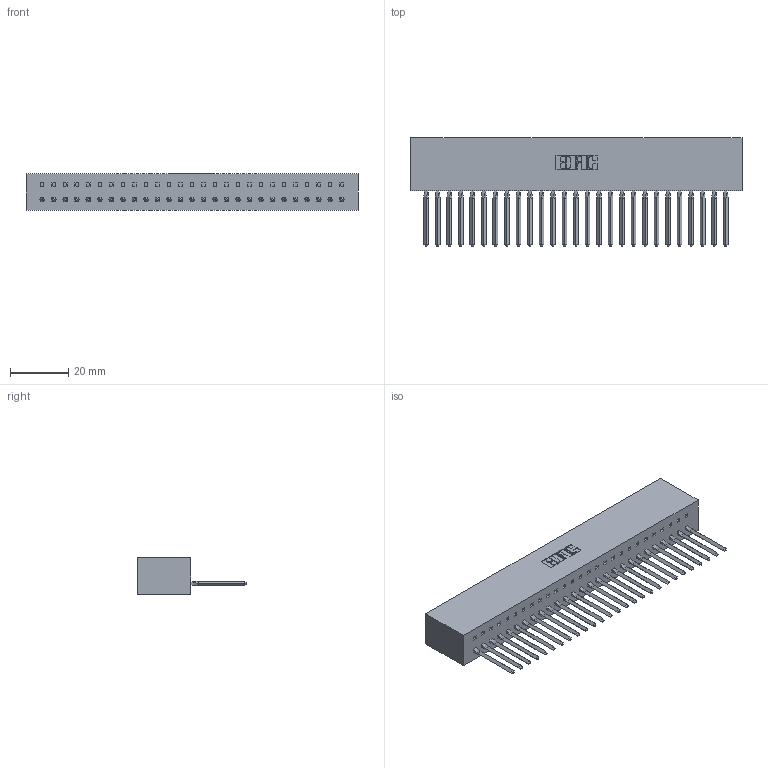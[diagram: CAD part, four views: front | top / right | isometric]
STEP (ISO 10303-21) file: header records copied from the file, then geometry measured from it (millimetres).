
FILE_DESCRIPTION (( 'STEP AP203' ), '1' );
FILE_NAME ('317-027-541-601.STEP', '2020-02-27T19:12:02', ( '' ), ( '' ), 'SwSTEP 2.0', 'SolidWorks 2016', '' );
FILE_SCHEMA (( 'CONFIG_CONTROL_DESIGN' ));
Length unit declared in the file: inch
Products named in the file (3): 317-290-002_541; 317 Part_Lugless; 317-027-541-601
Assembly tree (28 placements, depth 2):
  317-027-541-601
    317 Part_Lugless
    317-290-002_541  x27
Bounding box: 114.2 x 37.34 x 12.7 mm (x, y, z)
Volume: 19763.7 mm3; surface area: 27621.1 mm2
Topology: 28 solids, 28 shells, 4194 faces, 11957 edges, 7772 vertices
Faces by surface type: plane 3398, cylinder 688, bspline 108
Entity records: 41396 total; most frequent: CARTESIAN_POINT 7994, ORIENTED_EDGE 7274, DIRECTION 5955, EDGE_CURVE 3637, VECTOR 3281, LINE 3281, VERTEX_POINT 2416, AXIS2_PLACEMENT_3D 1337
